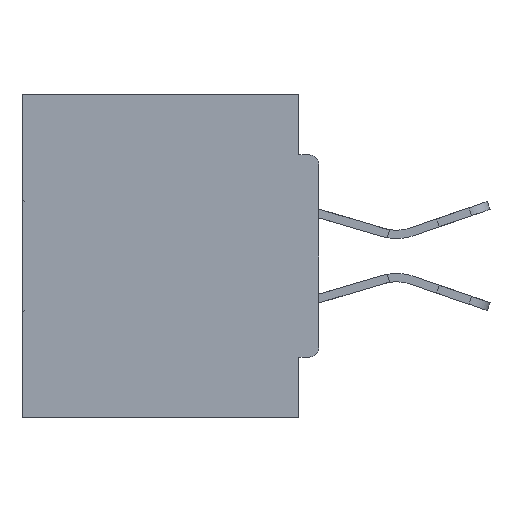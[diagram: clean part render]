
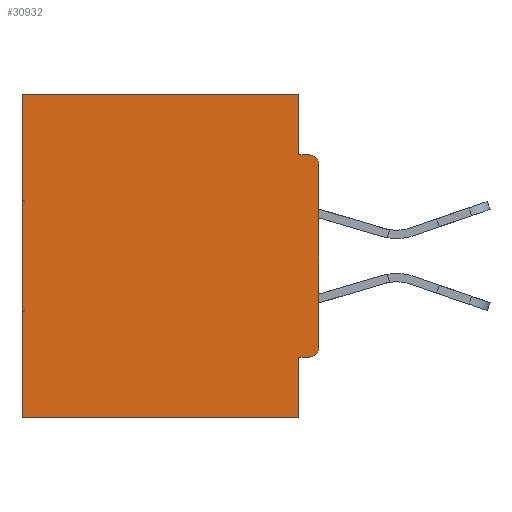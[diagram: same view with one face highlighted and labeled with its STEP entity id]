
A CAD part, left-side view. The second image highlights one B-rep face of the part: STEP entity #30932.
In plain terms, the highlighted planar face has unit normal (-1, 0, 0).
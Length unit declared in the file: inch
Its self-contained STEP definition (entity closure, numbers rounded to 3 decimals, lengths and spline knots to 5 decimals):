
#1465 = CARTESIAN_POINT ( 'NONE',  ( 0.298, 0., -0.4065 ) ) ;
#1502 = ORIENTED_EDGE ( 'NONE', *, *, #4629, .F. ) ;
#1989 = VECTOR ( 'NONE', #23624, 39.37008 ) ;
#2774 = EDGE_CURVE ( 'NONE', #29355, #9368, #40543, .T. ) ;
#4443 = CARTESIAN_POINT ( 'NONE',  ( 0.298, 0.015, -0.1085 ) ) ;
#4629 = EDGE_CURVE ( 'NONE', #28748, #43006, #22087, .T. ) ;
#4646 = CARTESIAN_POINT ( 'NONE',  ( 0.298, 0.031, -0.5 ) ) ;
#5413 = DIRECTION ( 'NONE',  ( 0., 1., 0. ) ) ;
#6981 = ORIENTED_EDGE ( 'NONE', *, *, #44018, .F. ) ;
#7274 = LINE ( 'NONE', #28076, #30488 ) ;
#7632 = DIRECTION ( 'NONE',  ( 0., 0., -1. ) ) ;
#8193 = DIRECTION ( 'NONE',  ( 0., 1., 0. ) ) ;
#8201 = DIRECTION ( 'NONE',  ( -1., 0., 0. ) ) ;
#9368 = VERTEX_POINT ( 'NONE', #21739 ) ;
#10709 = DIRECTION ( 'NONE',  ( 0., 0., -1. ) ) ;
#11045 = CIRCLE ( 'NONE', #35604, 0.015 ) ;
#11190 = ORIENTED_EDGE ( 'NONE', *, *, #26384, .F. ) ;
#11251 = ORIENTED_EDGE ( 'NONE', *, *, #12055, .T. ) ;
#11377 = ORIENTED_EDGE ( 'NONE', *, *, #2774, .F. ) ;
#11595 = CARTESIAN_POINT ( 'NONE',  ( 0.298, 0.46, 0. ) ) ;
#11884 = DIRECTION ( 'NONE',  ( 0., 0., -1. ) ) ;
#12055 = EDGE_CURVE ( 'NONE', #36803, #18119, #24166, .T. ) ;
#12552 = EDGE_CURVE ( 'NONE', #29355, #43006, #13272, .T. ) ;
#13272 = CIRCLE ( 'NONE', #14710, 0.015 ) ;
#13352 = VECTOR ( 'NONE', #5413, 39.37008 ) ;
#14053 = ORIENTED_EDGE ( 'NONE', *, *, #43425, .T. ) ;
#14639 = CARTESIAN_POINT ( 'NONE',  ( 0.298, 0.031, -0.5 ) ) ;
#14710 = AXIS2_PLACEMENT_3D ( 'NONE', #4443, #8201, #7632 ) ;
#15053 = LINE ( 'NONE', #14639, #25348 ) ;
#15710 = VECTOR ( 'NONE', #11884, 39.37008 ) ;
#15996 = CARTESIAN_POINT ( 'NONE',  ( 0.298, 0.031, -0.5 ) ) ;
#16036 = LINE ( 'NONE', #1465, #13352 ) ;
#16162 = ORIENTED_EDGE ( 'NONE', *, *, #33804, .F. ) ;
#16397 = CARTESIAN_POINT ( 'NONE',  ( 0.298, 0.031, 0. ) ) ;
#16473 = DIRECTION ( 'NONE',  ( 0., 0., -1. ) ) ;
#18105 = EDGE_CURVE ( 'NONE', #39618, #28748, #15053, .T. ) ;
#18119 = VERTEX_POINT ( 'NONE', #42613 ) ;
#19262 = CARTESIAN_POINT ( 'NONE',  ( 0.298, 0., -0.0935 ) ) ;
#19292 = AXIS2_PLACEMENT_3D ( 'NONE', #33424, #19667, #16473 ) ;
#19667 = DIRECTION ( 'NONE',  ( 1., 0., 0. ) ) ;
#20898 = CARTESIAN_POINT ( 'NONE',  ( 0.298, 0., -0.5 ) ) ;
#21282 = EDGE_CURVE ( 'NONE', #39618, #36803, #7274, .T. ) ;
#21739 = CARTESIAN_POINT ( 'NONE',  ( 0.298, 0., -0.3915 ) ) ;
#22087 = LINE ( 'NONE', #19262, #1989 ) ;
#22395 = CARTESIAN_POINT ( 'NONE',  ( 0.298, 0.031, -0.0935 ) ) ;
#22634 = DIRECTION ( 'NONE',  ( 0., 0., -1. ) ) ;
#23624 = DIRECTION ( 'NONE',  ( 0., -1., 0. ) ) ;
#24166 = LINE ( 'NONE', #11595, #41459 ) ;
#24681 = CARTESIAN_POINT ( 'NONE',  ( 0.298, 0., -0.1085 ) ) ;
#24940 = ORIENTED_EDGE ( 'NONE', *, *, #21282, .T. ) ;
#25090 = LINE ( 'NONE', #4646, #26629 ) ;
#25094 = DIRECTION ( 'NONE',  ( -1., 0., 0. ) ) ;
#25348 = VECTOR ( 'NONE', #35655, 39.37008 ) ;
#26342 = VERTEX_POINT ( 'NONE', #15996 ) ;
#26384 = EDGE_CURVE ( 'NONE', #26342, #18119, #36451, .T. ) ;
#26388 = ORIENTED_EDGE ( 'NONE', *, *, #18105, .F. ) ;
#26629 = VECTOR ( 'NONE', #32296, 39.37008 ) ;
#27935 = CARTESIAN_POINT ( 'NONE',  ( 0.298, 0.031, -0.4065 ) ) ;
#28076 = CARTESIAN_POINT ( 'NONE',  ( 0.298, 0., 0. ) ) ;
#28212 = EDGE_LOOP ( 'NONE', ( #28514, #1502, #26388, #24940, #11251, #11190, #6981, #16162, #14053, #11377 ) ) ;
#28402 = CARTESIAN_POINT ( 'NONE',  ( 0.298, 0.015, -0.3915 ) ) ;
#28514 = ORIENTED_EDGE ( 'NONE', *, *, #12552, .T. ) ;
#28748 = VERTEX_POINT ( 'NONE', #22395 ) ;
#29355 = VERTEX_POINT ( 'NONE', #24681 ) ;
#29695 = CARTESIAN_POINT ( 'NONE',  ( 0.298, 0., 0. ) ) ;
#29860 = FACE_OUTER_BOUND ( 'NONE', #28212, .T. ) ;
#30488 = VECTOR ( 'NONE', #8193, 39.37008 ) ;
#30932 = ADVANCED_FACE ( 'NONE', ( #29860 ), #37349, .F. ) ;
#31837 = DIRECTION ( 'NONE',  ( 0., 1., 0. ) ) ;
#32029 = CARTESIAN_POINT ( 'NONE',  ( 0.298, 0.46, 0. ) ) ;
#32296 = DIRECTION ( 'NONE',  ( 0., 0., -1. ) ) ;
#33424 = CARTESIAN_POINT ( 'NONE',  ( 0.298, 0., 0. ) ) ;
#33804 = EDGE_CURVE ( 'NONE', #37128, #44160, #16036, .T. ) ;
#35604 = AXIS2_PLACEMENT_3D ( 'NONE', #28402, #25094, #10709 ) ;
#35655 = DIRECTION ( 'NONE',  ( 0., 0., -1. ) ) ;
#36451 = LINE ( 'NONE', #20898, #43479 ) ;
#36803 = VERTEX_POINT ( 'NONE', #32029 ) ;
#37128 = VERTEX_POINT ( 'NONE', #40392 ) ;
#37349 = PLANE ( 'NONE',  #19292 ) ;
#39618 = VERTEX_POINT ( 'NONE', #16397 ) ;
#40392 = CARTESIAN_POINT ( 'NONE',  ( 0.298, 0.015, -0.4065 ) ) ;
#40543 = LINE ( 'NONE', #29695, #15710 ) ;
#41459 = VECTOR ( 'NONE', #22634, 39.37008 ) ;
#42613 = CARTESIAN_POINT ( 'NONE',  ( 0.298, 0.46, -0.5 ) ) ;
#43006 = VERTEX_POINT ( 'NONE', #43601 ) ;
#43425 = EDGE_CURVE ( 'NONE', #37128, #9368, #11045, .T. ) ;
#43479 = VECTOR ( 'NONE', #31837, 39.37008 ) ;
#43601 = CARTESIAN_POINT ( 'NONE',  ( 0.298, 0.015, -0.0935 ) ) ;
#44018 = EDGE_CURVE ( 'NONE', #44160, #26342, #25090, .T. ) ;
#44160 = VERTEX_POINT ( 'NONE', #27935 ) ;
